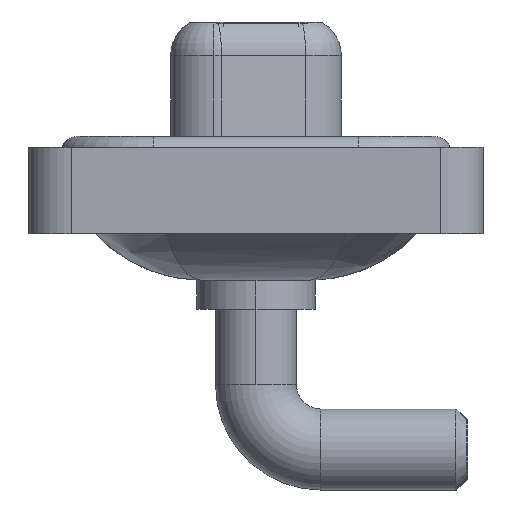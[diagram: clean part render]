
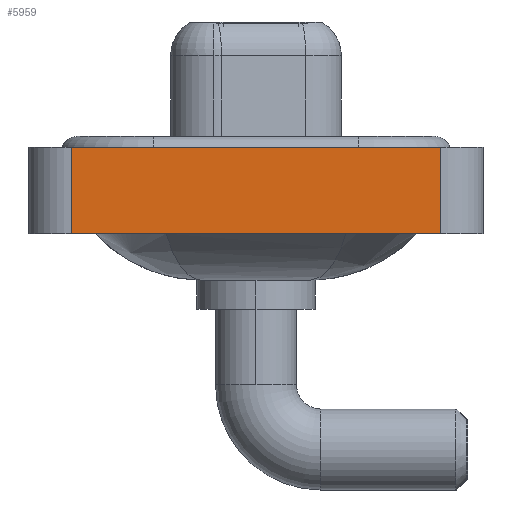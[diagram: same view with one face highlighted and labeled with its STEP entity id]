
A CAD part, left-side view. The second image highlights one B-rep face of the part: STEP entity #5959.
In plain terms, the highlighted planar face has unit normal (-1, 0, 0).
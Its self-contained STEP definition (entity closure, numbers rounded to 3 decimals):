
#155 = VERTEX_POINT ( 'NONE', #3381 ) ;
#658 = LINE ( 'NONE', #11367, #2601 ) ;
#682 = DIRECTION ( 'NONE',  ( 0., 0., 1. ) ) ;
#742 = EDGE_LOOP ( 'NONE', ( #15361, #13676, #5587, #1771 ) ) ;
#1771 = ORIENTED_EDGE ( 'NONE', *, *, #11973, .T. ) ;
#2601 = VECTOR ( 'NONE', #5916, 1000. ) ;
#3183 = LINE ( 'NONE', #15976, #5630 ) ;
#3381 = CARTESIAN_POINT ( 'NONE',  ( -7.3, 8.55, 0.4 ) ) ;
#3665 = VECTOR ( 'NONE', #5614, 1000. ) ;
#4052 = VERTEX_POINT ( 'NONE', #9843 ) ;
#4460 = DIRECTION ( 'NONE',  ( 0., -1., 0. ) ) ;
#4465 = LINE ( 'NONE', #9656, #3665 ) ;
#4799 = FACE_OUTER_BOUND ( 'NONE', #742, .T. ) ;
#4973 = PLANE ( 'NONE',  #6766 ) ;
#5531 = EDGE_CURVE ( 'NONE', #4052, #12987, #3183, .T. ) ;
#5587 = ORIENTED_EDGE ( 'NONE', *, *, #5822, .F. ) ;
#5614 = DIRECTION ( 'NONE',  ( 0., 0., 1. ) ) ;
#5630 = VECTOR ( 'NONE', #7218, 1000. ) ;
#5822 = EDGE_CURVE ( 'NONE', #9789, #155, #4465, .T. ) ;
#5916 = DIRECTION ( 'NONE',  ( 0., -1., 0. ) ) ;
#5959 = ADVANCED_FACE ( 'NONE', ( #4799 ), #4973, .T. ) ;
#6766 = AXIS2_PLACEMENT_3D ( 'NONE', #12984, #12810, #682 ) ;
#6777 = CARTESIAN_POINT ( 'NONE',  ( -7.3, 8.55, -3.6 ) ) ;
#7218 = DIRECTION ( 'NONE',  ( 0., 0., 1. ) ) ;
#9656 = CARTESIAN_POINT ( 'NONE',  ( -7.3, 8.55, -3.6 ) ) ;
#9789 = VERTEX_POINT ( 'NONE', #6777 ) ;
#9843 = CARTESIAN_POINT ( 'NONE',  ( -7.3, -8.55, -3.6 ) ) ;
#11127 = CARTESIAN_POINT ( 'NONE',  ( -7.3, -8.55, -3.6 ) ) ;
#11367 = CARTESIAN_POINT ( 'NONE',  ( -7.3, -8.55, 0.4 ) ) ;
#11973 = EDGE_CURVE ( 'NONE', #9789, #4052, #16339, .T. ) ;
#12810 = DIRECTION ( 'NONE',  ( -1., 0., 0. ) ) ;
#12984 = CARTESIAN_POINT ( 'NONE',  ( -7.3, -8.55, -3.6 ) ) ;
#12987 = VERTEX_POINT ( 'NONE', #16605 ) ;
#13676 = ORIENTED_EDGE ( 'NONE', *, *, #14011, .F. ) ;
#14011 = EDGE_CURVE ( 'NONE', #155, #12987, #658, .T. ) ;
#15361 = ORIENTED_EDGE ( 'NONE', *, *, #5531, .T. ) ;
#15976 = CARTESIAN_POINT ( 'NONE',  ( -7.3, -8.55, -3.6 ) ) ;
#16339 = LINE ( 'NONE', #11127, #16801 ) ;
#16605 = CARTESIAN_POINT ( 'NONE',  ( -7.3, -8.55, 0.4 ) ) ;
#16801 = VECTOR ( 'NONE', #4460, 1000. ) ;
